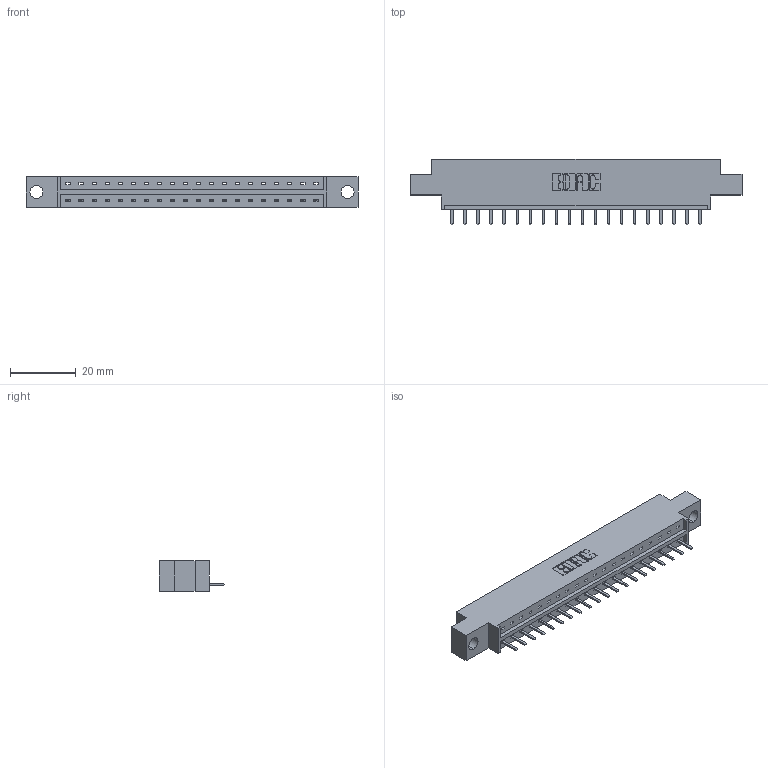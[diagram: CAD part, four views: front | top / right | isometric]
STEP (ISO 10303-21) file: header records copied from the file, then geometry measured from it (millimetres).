
FILE_DESCRIPTION (( 'STEP AP203' ), '1' );
FILE_NAME ('833-020-520-604.STEP', '2020-06-01T01:32:58', ( '' ), ( '' ), 'SwSTEP 2.0', 'SolidWorks 2020', '' );
FILE_SCHEMA (( 'CONFIG_CONTROL_DESIGN' ));
Length unit declared in the file: inch
Products named in the file (3): 345-292-001_345-293-120; 833 Part_Offset - .156 Dia - TH; 833-020-520-604
Assembly tree (21 placements, depth 2):
  833-020-520-604
    833 Part_Offset - .156 Dia - TH
    345-292-001_345-293-120  x20
Bounding box: 100.79 x 20.02 x 9.4 mm (x, y, z)
Volume: 9579.7 mm3; surface area: 10012.6 mm2
Topology: 21 solids, 21 shells, 1358 faces, 4003 edges, 2614 vertices
Faces by surface type: plane 954, cylinder 404
Entity records: 15321 total; most frequent: CARTESIAN_POINT 2666, ORIENTED_EDGE 2610, DIRECTION 2281, EDGE_CURVE 1305, LINE 1173, VECTOR 1173, VERTEX_POINT 866, AXIS2_PLACEMENT_3D 554
